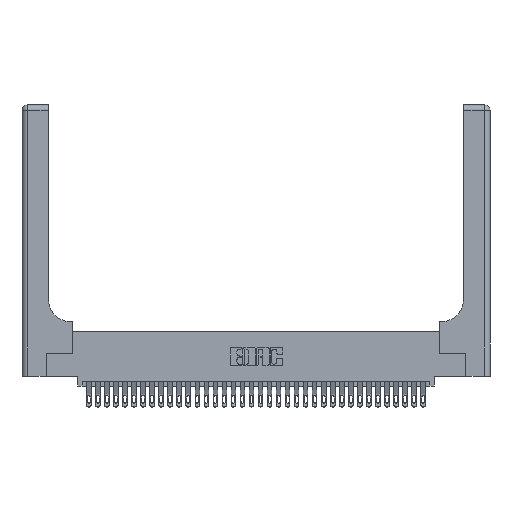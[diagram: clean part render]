
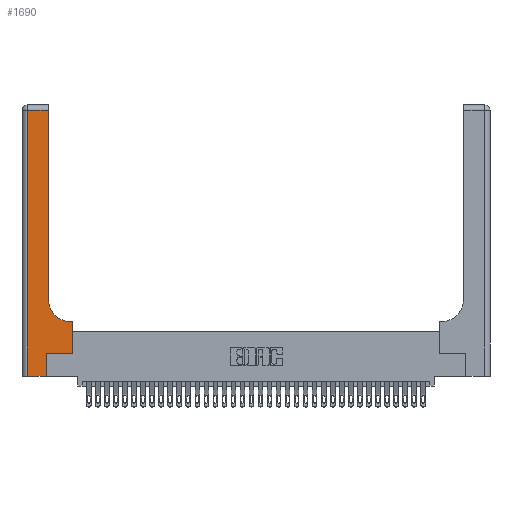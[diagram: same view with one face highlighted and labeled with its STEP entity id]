
A CAD part, top view. The second image highlights one B-rep face of the part: STEP entity #1690.
In plain terms, the highlighted planar face has unit normal (0, 0, 1).
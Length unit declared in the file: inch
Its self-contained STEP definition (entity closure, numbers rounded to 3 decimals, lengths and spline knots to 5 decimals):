
#369 = DIRECTION ( 'NONE',  ( -1., 0., 0. ) ) ;
#1171 = LINE ( 'NONE', #12869, #14265 ) ;
#1690 = ADVANCED_FACE ( 'NONE', ( #31522 ), #19741, .F. ) ;
#2455 = DIRECTION ( 'NONE',  ( 0., 1., 0. ) ) ;
#2684 = DIRECTION ( 'NONE',  ( 1., 0., 0. ) ) ;
#3088 = VECTOR ( 'NONE', #2455, 39.37008 ) ;
#3898 = CARTESIAN_POINT ( 'NONE',  ( 0.5415, 0.6, 0.37 ) ) ;
#3999 = LINE ( 'NONE', #16344, #3088 ) ;
#4489 = CARTESIAN_POINT ( 'NONE',  ( 0.5585, 0.25, 0.37 ) ) ;
#4928 = CARTESIAN_POINT ( 'NONE',  ( 0.5585, 0.25, 0.37 ) ) ;
#4934 = VERTEX_POINT ( 'NONE', #4489 ) ;
#6255 = CARTESIAN_POINT ( 'NONE',  ( 0.06, 0., 0.37 ) ) ;
#6386 = LINE ( 'NONE', #13283, #35913 ) ;
#7207 = ORIENTED_EDGE ( 'NONE', *, *, #7316, .T. ) ;
#7272 = EDGE_CURVE ( 'NONE', #27926, #12011, #20191, .T. ) ;
#7316 = EDGE_CURVE ( 'NONE', #22122, #26896, #24096, .T. ) ;
#7630 = EDGE_CURVE ( 'NONE', #4934, #22122, #14510, .T. ) ;
#8613 = VERTEX_POINT ( 'NONE', #9687 ) ;
#9304 = VECTOR ( 'NONE', #31524, 39.37008 ) ;
#9687 = CARTESIAN_POINT ( 'NONE',  ( 0.2915, 0.85, 0.37 ) ) ;
#10061 = AXIS2_PLACEMENT_3D ( 'NONE', #25328, #17068, #369 ) ;
#11054 = VECTOR ( 'NONE', #20141, 39.37008 ) ;
#11103 = ORIENTED_EDGE ( 'NONE', *, *, #17646, .T. ) ;
#11757 = CARTESIAN_POINT ( 'NONE',  ( 0., 0., 0.37 ) ) ;
#12011 = VERTEX_POINT ( 'NONE', #25409 ) ;
#12290 = ORIENTED_EDGE ( 'NONE', *, *, #29570, .T. ) ;
#12869 = CARTESIAN_POINT ( 'NONE',  ( 0.06, 3., 0.37 ) ) ;
#13283 = CARTESIAN_POINT ( 'NONE',  ( 0.2915, 3., 0.37 ) ) ;
#13682 = ORIENTED_EDGE ( 'NONE', *, *, #7272, .T. ) ;
#14247 = ORIENTED_EDGE ( 'NONE', *, *, #34468, .T. ) ;
#14265 = VECTOR ( 'NONE', #15671, 39.37008 ) ;
#14510 = LINE ( 'NONE', #4928, #35777 ) ;
#14686 = EDGE_LOOP ( 'NONE', ( #15717, #18248, #12290, #13682, #11103, #14247, #22636, #7207, #35102 ) ) ;
#15516 = VECTOR ( 'NONE', #22788, 39.37008 ) ;
#15671 = DIRECTION ( 'NONE',  ( 0., -1., 0. ) ) ;
#15717 = ORIENTED_EDGE ( 'NONE', *, *, #23546, .T. ) ;
#16079 = DIRECTION ( 'NONE',  ( 0., 1., 0. ) ) ;
#16344 = CARTESIAN_POINT ( 'NONE',  ( 0.269, 0., 0.37 ) ) ;
#17017 = CARTESIAN_POINT ( 'NONE',  ( 0.269, 0.25, 0.37 ) ) ;
#17065 = CARTESIAN_POINT ( 'NONE',  ( 0.269, 0.25, 0.37 ) ) ;
#17068 = DIRECTION ( 'NONE',  ( 0., 0., -1. ) ) ;
#17646 = EDGE_CURVE ( 'NONE', #12011, #20011, #3999, .T. ) ;
#17939 = DIRECTION ( 'NONE',  ( -1., 0., 0. ) ) ;
#17977 = CARTESIAN_POINT ( 'NONE',  ( 0.5585, 0.6, 0.37 ) ) ;
#18248 = ORIENTED_EDGE ( 'NONE', *, *, #20909, .T. ) ;
#18502 = CARTESIAN_POINT ( 'NONE',  ( 0.06, 2.94, 0.37 ) ) ;
#19374 = DIRECTION ( 'NONE',  ( 0., 0., -1. ) ) ;
#19741 = PLANE ( 'NONE',  #10061 ) ;
#20011 = VERTEX_POINT ( 'NONE', #17017 ) ;
#20141 = DIRECTION ( 'NONE',  ( 1., 0., 0. ) ) ;
#20191 = LINE ( 'NONE', #11757, #11054 ) ;
#20909 = EDGE_CURVE ( 'NONE', #22257, #27020, #33369, .T. ) ;
#22122 = VERTEX_POINT ( 'NONE', #17977 ) ;
#22257 = VERTEX_POINT ( 'NONE', #29101 ) ;
#22636 = ORIENTED_EDGE ( 'NONE', *, *, #7630, .T. ) ;
#22723 = CIRCLE ( 'NONE', #32977, 0.25 ) ;
#22788 = DIRECTION ( 'NONE',  ( 1., 0., 0. ) ) ;
#22911 = LINE ( 'NONE', #17065, #15516 ) ;
#23546 = EDGE_CURVE ( 'NONE', #8613, #22257, #6386, .T. ) ;
#24096 = LINE ( 'NONE', #25962, #9304 ) ;
#25328 = CARTESIAN_POINT ( 'NONE',  ( 0., 3., 0.37 ) ) ;
#25409 = CARTESIAN_POINT ( 'NONE',  ( 0.269, 0., 0.37 ) ) ;
#25962 = CARTESIAN_POINT ( 'NONE',  ( 0.2915, 0.6, 0.37 ) ) ;
#26896 = VERTEX_POINT ( 'NONE', #3898 ) ;
#27020 = VERTEX_POINT ( 'NONE', #18502 ) ;
#27926 = VERTEX_POINT ( 'NONE', #6255 ) ;
#29101 = CARTESIAN_POINT ( 'NONE',  ( 0.2915, 2.94, 0.37 ) ) ;
#29570 = EDGE_CURVE ( 'NONE', #27020, #27926, #1171, .T. ) ;
#30312 = EDGE_CURVE ( 'NONE', #26896, #8613, #22723, .T. ) ;
#31522 = FACE_OUTER_BOUND ( 'NONE', #14686, .T. ) ;
#31524 = DIRECTION ( 'NONE',  ( -1., 0., 0. ) ) ;
#31757 = CARTESIAN_POINT ( 'NONE',  ( 0., 2.94, 0.37 ) ) ;
#32485 = VECTOR ( 'NONE', #17939, 39.37008 ) ;
#32720 = DIRECTION ( 'NONE',  ( 0., 1., 0. ) ) ;
#32977 = AXIS2_PLACEMENT_3D ( 'NONE', #35973, #19374, #2684 ) ;
#33369 = LINE ( 'NONE', #31757, #32485 ) ;
#34468 = EDGE_CURVE ( 'NONE', #20011, #4934, #22911, .T. ) ;
#35102 = ORIENTED_EDGE ( 'NONE', *, *, #30312, .T. ) ;
#35777 = VECTOR ( 'NONE', #32720, 39.37008 ) ;
#35913 = VECTOR ( 'NONE', #16079, 39.37008 ) ;
#35973 = CARTESIAN_POINT ( 'NONE',  ( 0.5415, 0.85, 0.37 ) ) ;
